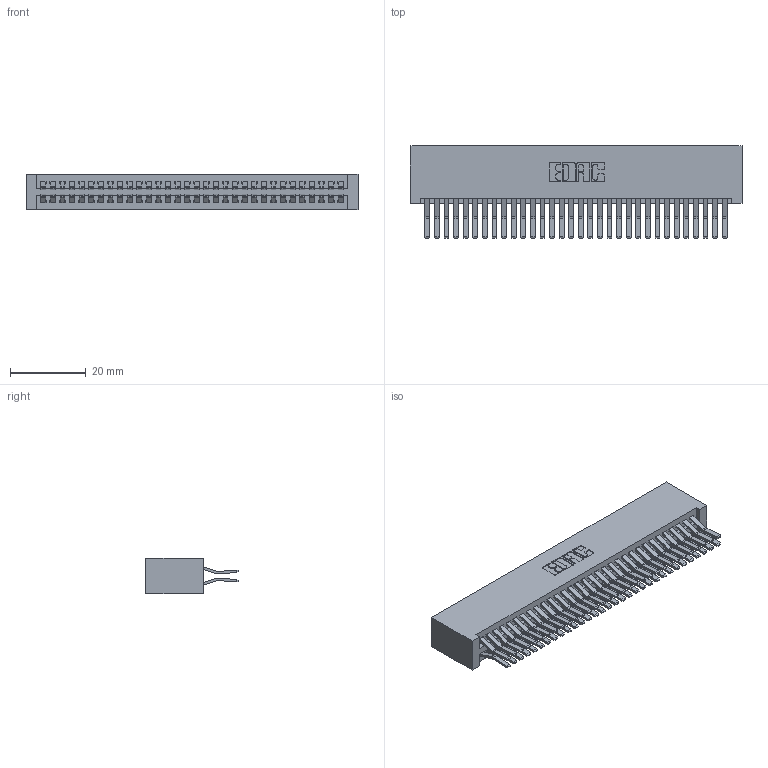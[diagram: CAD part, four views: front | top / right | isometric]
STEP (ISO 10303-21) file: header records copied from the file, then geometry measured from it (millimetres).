
FILE_DESCRIPTION (( 'STEP AP203' ), '1' );
FILE_NAME ('345-064-560-201.STEP', '2018-09-28T11:44:54', ( '' ), ( '' ), 'SwSTEP 2.0', 'SolidWorks 2016', '' );
FILE_SCHEMA (( 'CONFIG_CONTROL_DESIGN' ));
Length unit declared in the file: inch
Products named in the file (3): 345-064-560-201; 345-292-001_560 Tail; 345 Part_No Mounting Lugs
Assembly tree (65 placements, depth 2):
  345-064-560-201
    345 Part_No Mounting Lugs
    345-292-001_560 Tail  x64
Bounding box: 87.88 x 24.45 x 9.4 mm (x, y, z)
Volume: 9479.7 mm3; surface area: 15201.1 mm2
Topology: 65 solids, 65 shells, 3446 faces, 10237 edges, 6738 vertices
Faces by surface type: plane 2188, cylinder 1258
Entity records: 26265 total; most frequent: CARTESIAN_POINT 4412, ORIENTED_EDGE 4346, DIRECTION 3901, EDGE_CURVE 2173, VECTOR 1917, LINE 1917, VERTEX_POINT 1446, AXIS2_PLACEMENT_3D 992
